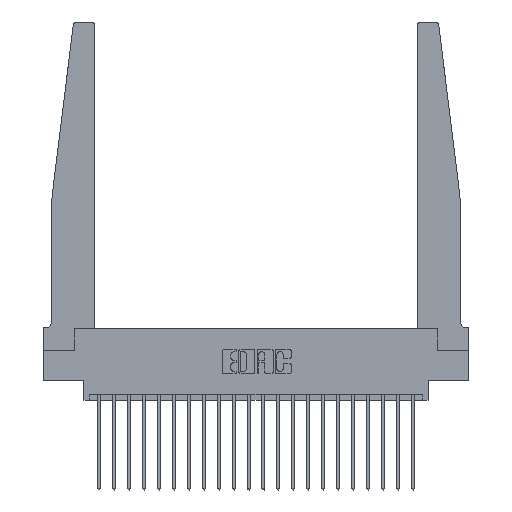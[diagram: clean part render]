
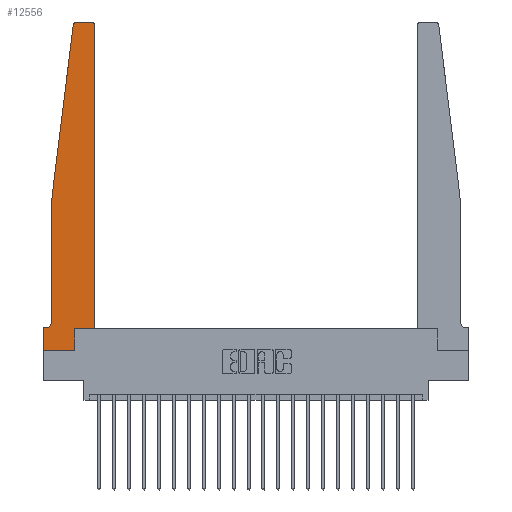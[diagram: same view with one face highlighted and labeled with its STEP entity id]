
A CAD part, top view. The second image highlights one B-rep face of the part: STEP entity #12556.
In plain terms, the highlighted planar face has unit normal (0, 0, 1).
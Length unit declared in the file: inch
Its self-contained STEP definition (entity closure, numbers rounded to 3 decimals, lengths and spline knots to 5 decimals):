
#319 = VECTOR ( 'NONE', #21369, 39.37008 ) ;
#361 = ORIENTED_EDGE ( 'NONE', *, *, #696, .T. ) ;
#696 = EDGE_CURVE ( 'NONE', #18882, #2439, #18288, .T. ) ;
#706 = ORIENTED_EDGE ( 'NONE', *, *, #15290, .T. ) ;
#952 = VERTEX_POINT ( 'NONE', #15976 ) ;
#1088 = CARTESIAN_POINT ( 'NONE',  ( 0., 0., 0.37 ) ) ;
#1095 = EDGE_CURVE ( 'NONE', #5988, #12494, #19744, .T. ) ;
#2209 = VECTOR ( 'NONE', #3327, 39.37008 ) ;
#2302 = DIRECTION ( 'NONE',  ( -1., 0., 0. ) ) ;
#2392 = DIRECTION ( 'NONE',  ( 1., 0., 0. ) ) ;
#2439 = VERTEX_POINT ( 'NONE', #2538 ) ;
#2538 = CARTESIAN_POINT ( 'NONE',  ( 0.27653, 2.75, 0.37 ) ) ;
#2596 = VECTOR ( 'NONE', #2302, 39.37008 ) ;
#2648 = CARTESIAN_POINT ( 'NONE',  ( 0.425, 0.18, 0.37 ) ) ;
#2875 = CARTESIAN_POINT ( 'NONE',  ( 0.425, 0.18, 0.37 ) ) ;
#3018 = ORIENTED_EDGE ( 'NONE', *, *, #20581, .T. ) ;
#3150 = CARTESIAN_POINT ( 'NONE',  ( 0., 0., 0.37 ) ) ;
#3188 = DIRECTION ( 'NONE',  ( 1., 0., 0. ) ) ;
#3327 = DIRECTION ( 'NONE',  ( 0., 1., 0. ) ) ;
#3994 = CARTESIAN_POINT ( 'NONE',  ( 0.065, 0.2375, 0.37 ) ) ;
#4101 = FACE_OUTER_BOUND ( 'NONE', #10179, .T. ) ;
#4590 = EDGE_CURVE ( 'NONE', #5978, #16381, #13611, .T. ) ;
#4680 = VERTEX_POINT ( 'NONE', #5802 ) ;
#5432 = CARTESIAN_POINT ( 'NONE',  ( 0.425, 2.72, 0.37 ) ) ;
#5802 = CARTESIAN_POINT ( 'NONE',  ( 0., 0., 0.37 ) ) ;
#5887 = CARTESIAN_POINT ( 'NONE',  ( 0.395, 2.75, 0.37 ) ) ;
#5922 = VECTOR ( 'NONE', #3188, 39.37008 ) ;
#5940 = EDGE_CURVE ( 'NONE', #2439, #12594, #14882, .T. ) ;
#5949 = CARTESIAN_POINT ( 'NONE',  ( 0., 0.1875, 0.37 ) ) ;
#5970 = DIRECTION ( 'NONE',  ( 0., 0., -1. ) ) ;
#5978 = VERTEX_POINT ( 'NONE', #7198 ) ;
#5988 = VERTEX_POINT ( 'NONE', #18062 ) ;
#6160 = CIRCLE ( 'NONE', #16266, 0.03 ) ;
#6223 = DIRECTION ( 'NONE',  ( 1., 0., 0. ) ) ;
#6252 = AXIS2_PLACEMENT_3D ( 'NONE', #6872, #13753, #17493 ) ;
#6612 = AXIS2_PLACEMENT_3D ( 'NONE', #10951, #5970, #21257 ) ;
#6627 = CIRCLE ( 'NONE', #6612, 0.05 ) ;
#6675 = ORIENTED_EDGE ( 'NONE', *, *, #15668, .T. ) ;
#6742 = EDGE_CURVE ( 'NONE', #952, #22050, #12739, .T. ) ;
#6872 = CARTESIAN_POINT ( 'NONE',  ( 0.27653, 2.72, 0.37 ) ) ;
#7198 = CARTESIAN_POINT ( 'NONE',  ( 0.2605, 0.18, 0.37 ) ) ;
#7488 = LINE ( 'NONE', #10996, #18814 ) ;
#7540 = CARTESIAN_POINT ( 'NONE',  ( 0.065, 0.1875, 0.37 ) ) ;
#7609 = VECTOR ( 'NONE', #12099, 39.37008 ) ;
#7952 = ORIENTED_EDGE ( 'NONE', *, *, #20259, .T. ) ;
#9470 = LINE ( 'NONE', #2648, #319 ) ;
#10179 = EDGE_LOOP ( 'NONE', ( #361, #11681, #706, #20004, #3018, #14354, #6675, #7952, #17496, #21877, #10993, #13281 ) ) ;
#10766 = DIRECTION ( 'NONE',  ( 1., 0., 0. ) ) ;
#10885 = DIRECTION ( 'NONE',  ( -0.122, -0.992, 0. ) ) ;
#10951 = CARTESIAN_POINT ( 'NONE',  ( 0.015, 0.2375, 0.37 ) ) ;
#10993 = ORIENTED_EDGE ( 'NONE', *, *, #15051, .T. ) ;
#10996 = CARTESIAN_POINT ( 'NONE',  ( 0.065, 1.25, 0.37 ) ) ;
#11342 = DIRECTION ( 'NONE',  ( 0., -1., 0. ) ) ;
#11444 = VERTEX_POINT ( 'NONE', #18828 ) ;
#11681 = ORIENTED_EDGE ( 'NONE', *, *, #5940, .T. ) ;
#12099 = DIRECTION ( 'NONE',  ( 0., -1., 0. ) ) ;
#12494 = VERTEX_POINT ( 'NONE', #3994 ) ;
#12556 = ADVANCED_FACE ( 'NONE', ( #4101 ), #14622, .T. ) ;
#12594 = VERTEX_POINT ( 'NONE', #18268 ) ;
#12739 = LINE ( 'NONE', #7540, #2596 ) ;
#12937 = CARTESIAN_POINT ( 'NONE',  ( 0., 0.1875, 0.37 ) ) ;
#13281 = ORIENTED_EDGE ( 'NONE', *, *, #15242, .T. ) ;
#13611 = LINE ( 'NONE', #18727, #5922 ) ;
#13753 = DIRECTION ( 'NONE',  ( 0., 0., 1. ) ) ;
#14354 = ORIENTED_EDGE ( 'NONE', *, *, #6742, .T. ) ;
#14622 = PLANE ( 'NONE',  #22351 ) ;
#14685 = LINE ( 'NONE', #1088, #15979 ) ;
#14882 = CIRCLE ( 'NONE', #6252, 0.03 ) ;
#15051 = EDGE_CURVE ( 'NONE', #16381, #18888, #9470, .T. ) ;
#15242 = EDGE_CURVE ( 'NONE', #18888, #18882, #6160, .T. ) ;
#15290 = EDGE_CURVE ( 'NONE', #12594, #5988, #7488, .T. ) ;
#15547 = CARTESIAN_POINT ( 'NONE',  ( 0.395, 2.72, 0.37 ) ) ;
#15668 = EDGE_CURVE ( 'NONE', #22050, #4680, #22206, .T. ) ;
#15976 = CARTESIAN_POINT ( 'NONE',  ( 0.015, 0.1875, 0.37 ) ) ;
#15979 = VECTOR ( 'NONE', #6223, 39.37008 ) ;
#16059 = VECTOR ( 'NONE', #11342, 39.37008 ) ;
#16266 = AXIS2_PLACEMENT_3D ( 'NONE', #15547, #18868, #10766 ) ;
#16322 = CARTESIAN_POINT ( 'NONE',  ( 0.065, 1.25, 0.37 ) ) ;
#16381 = VERTEX_POINT ( 'NONE', #2875 ) ;
#16810 = LINE ( 'NONE', #18870, #2209 ) ;
#17493 = DIRECTION ( 'NONE',  ( 1., 0., 0. ) ) ;
#17496 = ORIENTED_EDGE ( 'NONE', *, *, #19093, .T. ) ;
#17932 = DIRECTION ( 'NONE',  ( 0., 0., 1. ) ) ;
#18062 = CARTESIAN_POINT ( 'NONE',  ( 0.065, 1.25, 0.37 ) ) ;
#18268 = CARTESIAN_POINT ( 'NONE',  ( 0.24675, 2.72367, 0.37 ) ) ;
#18288 = LINE ( 'NONE', #20207, #20822 ) ;
#18515 = DIRECTION ( 'NONE',  ( -1., 0., 0. ) ) ;
#18727 = CARTESIAN_POINT ( 'NONE',  ( 0.425, 0.18, 0.37 ) ) ;
#18814 = VECTOR ( 'NONE', #10885, 39.37008 ) ;
#18828 = CARTESIAN_POINT ( 'NONE',  ( 0.2605, 0., 0.37 ) ) ;
#18868 = DIRECTION ( 'NONE',  ( 0., 0., 1. ) ) ;
#18870 = CARTESIAN_POINT ( 'NONE',  ( 0.2605, 0.18, 0.37 ) ) ;
#18882 = VERTEX_POINT ( 'NONE', #5887 ) ;
#18888 = VERTEX_POINT ( 'NONE', #5432 ) ;
#19093 = EDGE_CURVE ( 'NONE', #11444, #5978, #16810, .T. ) ;
#19744 = LINE ( 'NONE', #16322, #16059 ) ;
#20004 = ORIENTED_EDGE ( 'NONE', *, *, #1095, .T. ) ;
#20207 = CARTESIAN_POINT ( 'NONE',  ( 0.25, 2.75, 0.37 ) ) ;
#20259 = EDGE_CURVE ( 'NONE', #4680, #11444, #14685, .T. ) ;
#20581 = EDGE_CURVE ( 'NONE', #12494, #952, #6627, .T. ) ;
#20822 = VECTOR ( 'NONE', #18515, 39.37008 ) ;
#21257 = DIRECTION ( 'NONE',  ( -1., 0., 0. ) ) ;
#21369 = DIRECTION ( 'NONE',  ( 0., 1., 0. ) ) ;
#21877 = ORIENTED_EDGE ( 'NONE', *, *, #4590, .T. ) ;
#22050 = VERTEX_POINT ( 'NONE', #5949 ) ;
#22206 = LINE ( 'NONE', #3150, #7609 ) ;
#22351 = AXIS2_PLACEMENT_3D ( 'NONE', #12937, #17932, #2392 ) ;
